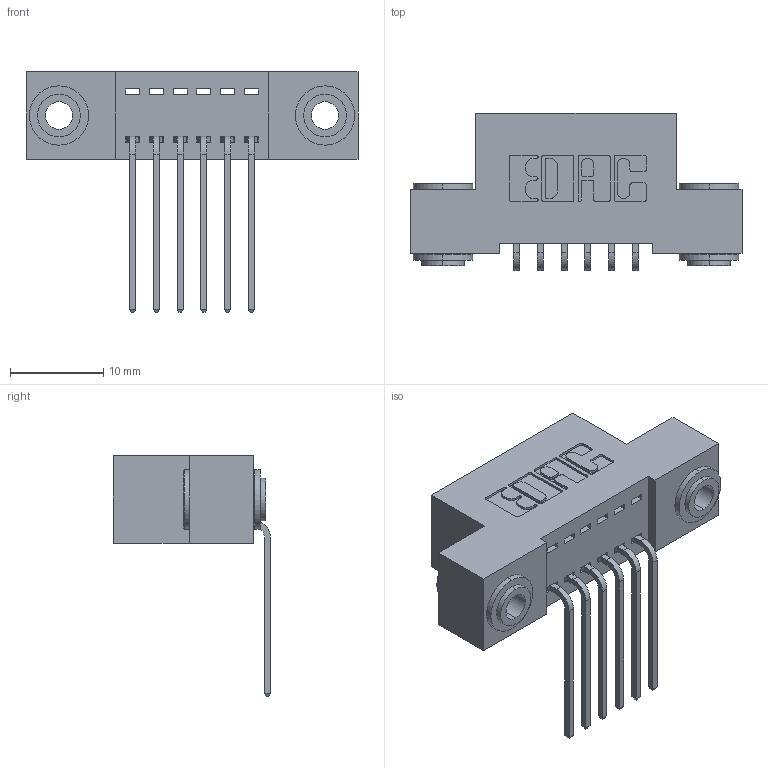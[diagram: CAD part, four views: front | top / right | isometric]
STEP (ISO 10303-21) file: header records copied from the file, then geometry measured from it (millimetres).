
FILE_DESCRIPTION (( 'STEP AP203' ), '1' );
FILE_NAME ('392-006-559-103.STEP', '2018-08-14T17:52:39', ( '' ), ( '' ), 'SwSTEP 2.0', 'SolidWorks 2016', '' );
FILE_SCHEMA (( 'CONFIG_CONTROL_DESIGN' ));
Length unit declared in the file: inch
Products named in the file (4): 392-006-559-103; 342 Part_.156 TH; 345-292-001_558 559 Tail - 1; 342-250-002_345-250-002-102
Assembly tree (9 placements, depth 2):
  392-006-559-103
    342 Part_.156 TH
    345-292-001_558 559 Tail - 1  x6
    342-250-002_345-250-002-102  x2
Bounding box: 35.56 x 16.83 x 25.78 mm (x, y, z)
Volume: 3028.1 mm3; surface area: 4114.2 mm2
Topology: 9 solids, 9 shells, 508 faces, 1467 edges, 966 vertices
Faces by surface type: plane 340, cylinder 160, cone 8
Entity records: 8926 total; most frequent: CARTESIAN_POINT 1523, ORIENTED_EDGE 1458, DIRECTION 1391, EDGE_CURVE 729, VECTOR 577, LINE 577, VERTEX_POINT 482, AXIS2_PLACEMENT_3D 407
